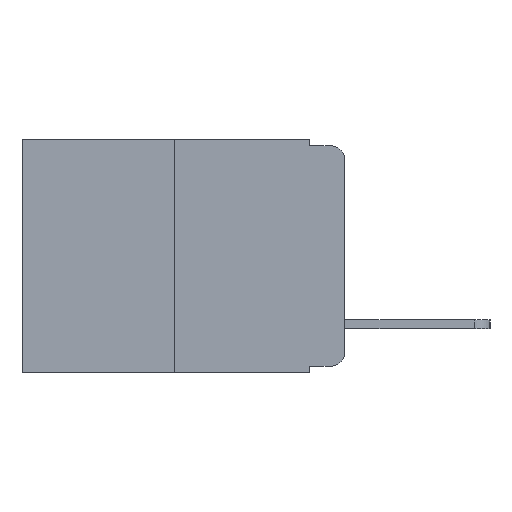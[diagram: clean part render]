
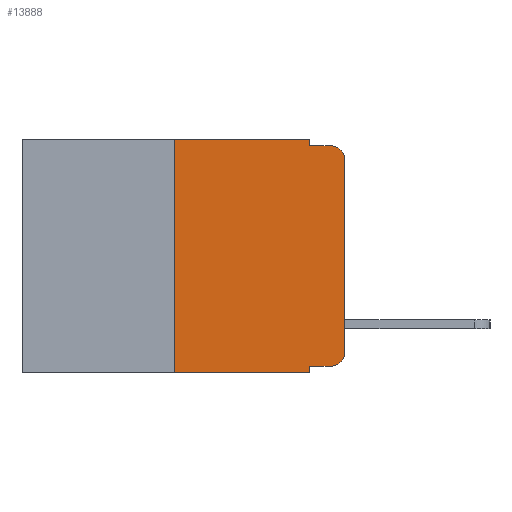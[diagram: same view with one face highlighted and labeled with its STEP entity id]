
A CAD part, left-side view. The second image highlights one B-rep face of the part: STEP entity #13888.
In plain terms, the highlighted planar face has unit normal (-1, 0, 0).
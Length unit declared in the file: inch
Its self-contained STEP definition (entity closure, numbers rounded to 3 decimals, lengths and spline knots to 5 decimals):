
#172 = ORIENTED_EDGE ( 'NONE', *, *, #5099, .T. ) ;
#215 = CIRCLE ( 'NONE', #16231, 0.02 ) ;
#226 = EDGE_LOOP ( 'NONE', ( #20531, #172, #2355, #5455, #4532, #13981, #2701, #1146, #7736, #264 ) ) ;
#264 = ORIENTED_EDGE ( 'NONE', *, *, #10254, .T. ) ;
#343 = CARTESIAN_POINT ( 'NONE',  ( 0., 0.02, -0.333 ) ) ;
#1146 = ORIENTED_EDGE ( 'NONE', *, *, #19981, .F. ) ;
#1266 = LINE ( 'NONE', #8497, #11775 ) ;
#1562 = VERTEX_POINT ( 'NONE', #10398 ) ;
#2111 = EDGE_CURVE ( 'NONE', #2501, #17585, #17594, .T. ) ;
#2146 = VECTOR ( 'NONE', #6440, 39.37008 ) ;
#2355 = ORIENTED_EDGE ( 'NONE', *, *, #19837, .F. ) ;
#2501 = VERTEX_POINT ( 'NONE', #5930 ) ;
#2701 = ORIENTED_EDGE ( 'NONE', *, *, #14256, .T. ) ;
#2842 = VECTOR ( 'NONE', #6921, 39.37008 ) ;
#3322 = CARTESIAN_POINT ( 'NONE',  ( 0., 0.473, 0. ) ) ;
#4059 = LINE ( 'NONE', #18419, #8735 ) ;
#4532 = ORIENTED_EDGE ( 'NONE', *, *, #11178, .F. ) ;
#4693 = VECTOR ( 'NONE', #12337, 39.37008 ) ;
#4900 = CARTESIAN_POINT ( 'NONE',  ( 0., 0.051, 0. ) ) ;
#5099 = EDGE_CURVE ( 'NONE', #7631, #24279, #22092, .T. ) ;
#5307 = PLANE ( 'NONE',  #14281 ) ;
#5372 = CARTESIAN_POINT ( 'NONE',  ( 0., 0.25, 0. ) ) ;
#5455 = ORIENTED_EDGE ( 'NONE', *, *, #17688, .F. ) ;
#5930 = CARTESIAN_POINT ( 'NONE',  ( 0., 0.25, -0.343 ) ) ;
#6440 = DIRECTION ( 'NONE',  ( 0., 0., 1. ) ) ;
#6489 = DIRECTION ( 'NONE',  ( 0., -1., 0. ) ) ;
#6630 = VECTOR ( 'NONE', #10084, 39.37008 ) ;
#6919 = DIRECTION ( 'NONE',  ( 0., -1., 0. ) ) ;
#6921 = DIRECTION ( 'NONE',  ( 0., 0., -1. ) ) ;
#6998 = CARTESIAN_POINT ( 'NONE',  ( 0., 0.02, -0.313 ) ) ;
#7000 = VERTEX_POINT ( 'NONE', #343 ) ;
#7597 = EDGE_CURVE ( 'NONE', #24658, #7000, #1266, .T. ) ;
#7631 = VERTEX_POINT ( 'NONE', #10554 ) ;
#7711 = AXIS2_PLACEMENT_3D ( 'NONE', #9469, #22887, #11392 ) ;
#7736 = ORIENTED_EDGE ( 'NONE', *, *, #7597, .T. ) ;
#8152 = FACE_OUTER_BOUND ( 'NONE', #226, .T. ) ;
#8156 = LINE ( 'NONE', #4900, #2842 ) ;
#8497 = CARTESIAN_POINT ( 'NONE',  ( 0., 0.051, -0.333 ) ) ;
#8735 = VECTOR ( 'NONE', #6919, 39.37008 ) ;
#9014 = DIRECTION ( 'NONE',  ( 0., 0., -1. ) ) ;
#9469 = CARTESIAN_POINT ( 'NONE',  ( 0., 0.02, -0.03 ) ) ;
#9847 = CARTESIAN_POINT ( 'NONE',  ( 0., 0.473, 0. ) ) ;
#10073 = CARTESIAN_POINT ( 'NONE',  ( 0., 0.02, -0.01 ) ) ;
#10084 = DIRECTION ( 'NONE',  ( 0., 0., 1. ) ) ;
#10130 = LINE ( 'NONE', #9847, #19023 ) ;
#10254 = EDGE_CURVE ( 'NONE', #7000, #20100, #215, .T. ) ;
#10398 = CARTESIAN_POINT ( 'NONE',  ( 0., 0.051, -0.343 ) ) ;
#10554 = CARTESIAN_POINT ( 'NONE',  ( 0., 0., -0.03 ) ) ;
#11178 = EDGE_CURVE ( 'NONE', #17585, #23829, #10130, .T. ) ;
#11271 = DIRECTION ( 'NONE',  ( 0., 0., -1. ) ) ;
#11392 = DIRECTION ( 'NONE',  ( 0., 0., -1. ) ) ;
#11750 = DIRECTION ( 'NONE',  ( 0., 0., -1. ) ) ;
#11775 = VECTOR ( 'NONE', #6489, 39.37008 ) ;
#12337 = DIRECTION ( 'NONE',  ( 0., -1., 0. ) ) ;
#12939 = EDGE_CURVE ( 'NONE', #20100, #7631, #21435, .T. ) ;
#13888 = ADVANCED_FACE ( 'NONE', ( #8152 ), #5307, .F. ) ;
#13941 = VECTOR ( 'NONE', #11750, 39.37008 ) ;
#13981 = ORIENTED_EDGE ( 'NONE', *, *, #2111, .F. ) ;
#14256 = EDGE_CURVE ( 'NONE', #2501, #1562, #4059, .T. ) ;
#14281 = AXIS2_PLACEMENT_3D ( 'NONE', #3322, #22761, #11271 ) ;
#14360 = CARTESIAN_POINT ( 'NONE',  ( 0., 0.051, 0. ) ) ;
#16231 = AXIS2_PLACEMENT_3D ( 'NONE', #6998, #20450, #9014 ) ;
#17585 = VERTEX_POINT ( 'NONE', #22932 ) ;
#17594 = LINE ( 'NONE', #5372, #2146 ) ;
#17688 = EDGE_CURVE ( 'NONE', #23829, #20766, #19031, .T. ) ;
#18419 = CARTESIAN_POINT ( 'NONE',  ( 0., 0.473, -0.343 ) ) ;
#18751 = CARTESIAN_POINT ( 'NONE',  ( 0., 0., -0.313 ) ) ;
#19023 = VECTOR ( 'NONE', #19413, 39.37008 ) ;
#19031 = LINE ( 'NONE', #19348, #13941 ) ;
#19262 = CARTESIAN_POINT ( 'NONE',  ( 0., 0.051, -0.01 ) ) ;
#19348 = CARTESIAN_POINT ( 'NONE',  ( 0., 0.051, 0. ) ) ;
#19413 = DIRECTION ( 'NONE',  ( 0., -1., 0. ) ) ;
#19837 = EDGE_CURVE ( 'NONE', #20766, #24279, #20116, .T. ) ;
#19981 = EDGE_CURVE ( 'NONE', #24658, #1562, #8156, .T. ) ;
#20100 = VERTEX_POINT ( 'NONE', #18751 ) ;
#20116 = LINE ( 'NONE', #21947, #4693 ) ;
#20450 = DIRECTION ( 'NONE',  ( -1., 0., 0. ) ) ;
#20531 = ORIENTED_EDGE ( 'NONE', *, *, #12939, .T. ) ;
#20766 = VERTEX_POINT ( 'NONE', #19262 ) ;
#21435 = LINE ( 'NONE', #23491, #6630 ) ;
#21947 = CARTESIAN_POINT ( 'NONE',  ( 0., 0.051, -0.01 ) ) ;
#22092 = CIRCLE ( 'NONE', #7711, 0.02 ) ;
#22761 = DIRECTION ( 'NONE',  ( 1., 0., 0. ) ) ;
#22887 = DIRECTION ( 'NONE',  ( -1., 0., 0. ) ) ;
#22932 = CARTESIAN_POINT ( 'NONE',  ( 0., 0.25, 0. ) ) ;
#23491 = CARTESIAN_POINT ( 'NONE',  ( 0., 0., 0. ) ) ;
#23829 = VERTEX_POINT ( 'NONE', #14360 ) ;
#24279 = VERTEX_POINT ( 'NONE', #10073 ) ;
#24552 = CARTESIAN_POINT ( 'NONE',  ( 0., 0.051, -0.333 ) ) ;
#24658 = VERTEX_POINT ( 'NONE', #24552 ) ;
